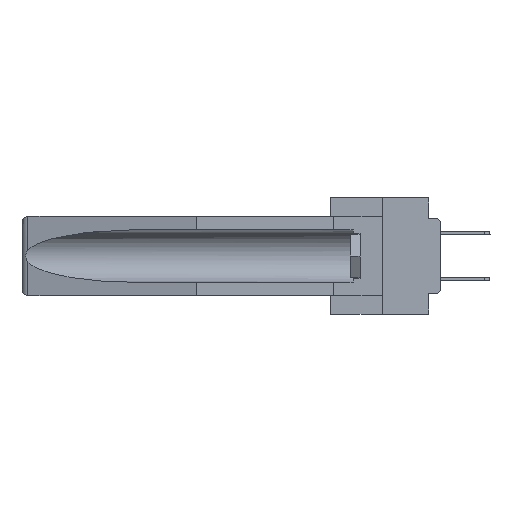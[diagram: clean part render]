
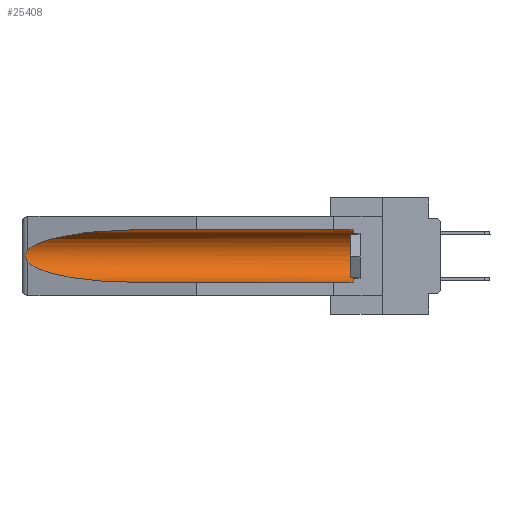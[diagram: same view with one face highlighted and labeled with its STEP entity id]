
A CAD part, left-side view. The second image highlights one B-rep face of the part: STEP entity #25408.
In plain terms, the highlighted cylindrical face has radius 2.857 mm (diameter 5.715 mm), a partial arc.
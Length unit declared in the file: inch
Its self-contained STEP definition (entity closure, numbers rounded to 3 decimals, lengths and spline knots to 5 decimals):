
#177 = EDGE_LOOP ( 'NONE', ( #36599, #20662, #4630, #12583, #23962, #25030 ) ) ;
#1125 = DIRECTION ( 'NONE',  ( 0., 1., 0. ) ) ;
#1772 = DIRECTION ( 'NONE',  ( 0., 1., 0. ) ) ;
#2267 = CARTESIAN_POINT ( 'NONE',  ( 0.26654, 1.53092, -0.15636 ) ) ;
#2300 = VERTEX_POINT ( 'NONE', #22745 ) ;
#2950 = EDGE_CURVE ( 'NONE', #25853, #2300, #19670, .T. ) ;
#4628 = EDGE_CURVE ( 'NONE', #18142, #21055, #12655, .T. ) ;
#4630 = ORIENTED_EDGE ( 'NONE', *, *, #11952, .T. ) ;
#4873 = CARTESIAN_POINT ( 'NONE',  ( 0.26597, 1.5296, -0.19026 ) ) ;
#4885 = CARTESIAN_POINT ( 'NONE',  ( 0.155, 1.07973, -0.059 ) ) ;
#5062 = CARTESIAN_POINT ( 'NONE',  ( 0.2675, 1.53308, -0.16763 ) ) ;
#6784 = CARTESIAN_POINT ( 'NONE',  ( 0.26537, 1.52718, -0.19328 ) ) ;
#7497 = CARTESIAN_POINT ( 'NONE',  ( 0.26655, 1.53094, -0.18657 ) ) ;
#8425 = CARTESIAN_POINT ( 'NONE',  ( 0.26537, 1.52718, -0.14972 ) ) ;
#8429 = AXIS2_PLACEMENT_3D ( 'NONE', #34625, #24493, #13179 ) ;
#9208 = CARTESIAN_POINT ( 'NONE',  ( 0.21114, 1.30732, -0.284 ) ) ;
#10803 = CARTESIAN_POINT ( 'NONE',  ( 0.155, 0.126, -0.284 ) ) ;
#11541 = CARTESIAN_POINT ( 'NONE',  ( 0.155, -0.30754, -0.059 ) ) ;
#11952 = EDGE_CURVE ( 'NONE', #21055, #31180, #20060, .T. ) ;
#12092 = LINE ( 'NONE', #11541, #16610 ) ;
#12490 = CARTESIAN_POINT ( 'NONE',  ( 0.155, -0.30754, -0.284 ) ) ;
#12583 = ORIENTED_EDGE ( 'NONE', *, *, #25661, .F. ) ;
#12655 = B_SPLINE_CURVE_WITH_KNOTS ( 'NONE', 3,
 ( #21605, #27912, #2267, #30557, #5062, #32970, #16402, #7497, #4873, #13618 ),
 .UNSPECIFIED., .F., .F.,
 ( 4, 2, 2, 2, 4 ),
 ( 0., 0.00029, 0.00058, 0.00087, 0.00117 ),
 .UNSPECIFIED. ) ;
#13121 = DIRECTION ( 'NONE',  ( 0., 0., 1. ) ) ;
#13179 = DIRECTION ( 'NONE',  ( 0., 0., 1. ) ) ;
#13618 = CARTESIAN_POINT ( 'NONE',  ( 0.26537, 1.52718, -0.19328 ) ) ;
#14186 = CARTESIAN_POINT ( 'NONE',  ( 0.25451, 1.48313, -0.09465 ) ) ;
#15278 = LINE ( 'NONE', #12490, #25751 ) ;
#15899 = CYLINDRICAL_SURFACE ( 'NONE', #35850, 0.1125 ) ;
#16402 = CARTESIAN_POINT ( 'NONE',  ( 0.2673, 1.53269, -0.17917 ) ) ;
#16610 = VECTOR ( 'NONE', #28993, 39.37008 ) ;
#16954 = CARTESIAN_POINT ( 'NONE',  ( 0.21114, 1.30732, -0.059 ) ) ;
#18142 = VERTEX_POINT ( 'NONE', #18927 ) ;
#18927 = CARTESIAN_POINT ( 'NONE',  ( 0.26537, 1.52718, -0.14972 ) ) ;
#19670 = CIRCLE ( 'NONE', #8429, 0.1125 ) ;
#20060 =( BOUNDED_CURVE ( )  B_SPLINE_CURVE ( 3, ( #6784, #20880, #9208, #20519 ),
 .UNSPECIFIED., .F., .F. ) 
 B_SPLINE_CURVE_WITH_KNOTS ( ( 4, 4 ),
 ( 0.1948, 1.5708 ),
 .UNSPECIFIED. ) 
 CURVE ( )  GEOMETRIC_REPRESENTATION_ITEM ( )  RATIONAL_B_SPLINE_CURVE ( ( 1., 0.848, 0.848, 1. ) ) 
 REPRESENTATION_ITEM ( '' )  );
#20519 = CARTESIAN_POINT ( 'NONE',  ( 0.155, 1.07973, -0.284 ) ) ;
#20662 = ORIENTED_EDGE ( 'NONE', *, *, #4628, .T. ) ;
#20880 = CARTESIAN_POINT ( 'NONE',  ( 0.25451, 1.48313, -0.24835 ) ) ;
#21055 = VERTEX_POINT ( 'NONE', #34128 ) ;
#21605 = CARTESIAN_POINT ( 'NONE',  ( 0.26537, 1.52718, -0.14972 ) ) ;
#22745 = CARTESIAN_POINT ( 'NONE',  ( 0.155, 0.126, -0.059 ) ) ;
#23121 = CARTESIAN_POINT ( 'NONE',  ( 0.155, 1.07973, -0.059 ) ) ;
#23545 = CARTESIAN_POINT ( 'NONE',  ( 0.155, 1.07973, -0.284 ) ) ;
#23962 = ORIENTED_EDGE ( 'NONE', *, *, #2950, .T. ) ;
#24493 = DIRECTION ( 'NONE',  ( 0., -1., 0. ) ) ;
#25030 = ORIENTED_EDGE ( 'NONE', *, *, #33410, .T. ) ;
#25408 = ADVANCED_FACE ( 'NONE', ( #30063 ), #15899, .F. ) ;
#25661 = EDGE_CURVE ( 'NONE', #25853, #31180, #15278, .T. ) ;
#25751 = VECTOR ( 'NONE', #1125, 39.37008 ) ;
#25853 = VERTEX_POINT ( 'NONE', #10803 ) ;
#27231 = CARTESIAN_POINT ( 'NONE',  ( 0.155, -0.30754, -0.1715 ) ) ;
#27312 = EDGE_CURVE ( 'NONE', #28335, #18142, #36687, .T. ) ;
#27912 = CARTESIAN_POINT ( 'NONE',  ( 0.26597, 1.52961, -0.15275 ) ) ;
#28335 = VERTEX_POINT ( 'NONE', #23121 ) ;
#28993 = DIRECTION ( 'NONE',  ( 0., 1., 0. ) ) ;
#30063 = FACE_OUTER_BOUND ( 'NONE', #177, .T. ) ;
#30557 = CARTESIAN_POINT ( 'NONE',  ( 0.2673, 1.5327, -0.16383 ) ) ;
#31180 = VERTEX_POINT ( 'NONE', #23545 ) ;
#32970 = CARTESIAN_POINT ( 'NONE',  ( 0.2675, 1.53308, -0.17534 ) ) ;
#33410 = EDGE_CURVE ( 'NONE', #2300, #28335, #12092, .T. ) ;
#34128 = CARTESIAN_POINT ( 'NONE',  ( 0.26537, 1.52718, -0.19328 ) ) ;
#34625 = CARTESIAN_POINT ( 'NONE',  ( 0.155, 0.126, -0.1715 ) ) ;
#35850 = AXIS2_PLACEMENT_3D ( 'NONE', #27231, #1772, #13121 ) ;
#36599 = ORIENTED_EDGE ( 'NONE', *, *, #27312, .T. ) ;
#36687 =( BOUNDED_CURVE ( )  B_SPLINE_CURVE ( 3, ( #4885, #16954, #14186, #8425 ),
 .UNSPECIFIED., .F., .T. ) 
 B_SPLINE_CURVE_WITH_KNOTS ( ( 4, 4 ),
 ( 4.71239, 6.08839 ),
 .UNSPECIFIED. ) 
 CURVE ( )  GEOMETRIC_REPRESENTATION_ITEM ( )  RATIONAL_B_SPLINE_CURVE ( ( 1., 0.848, 0.848, 1. ) ) 
 REPRESENTATION_ITEM ( '' )  );
